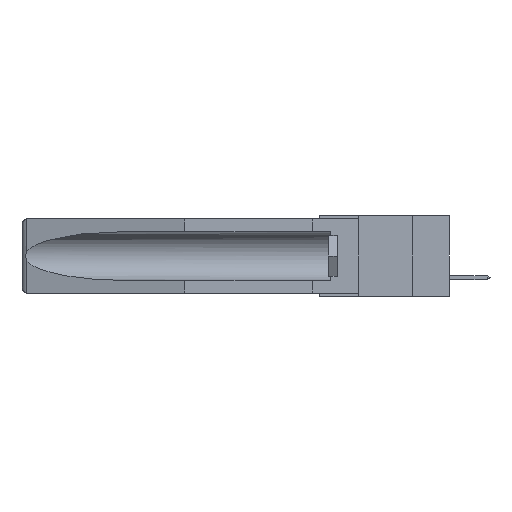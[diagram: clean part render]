
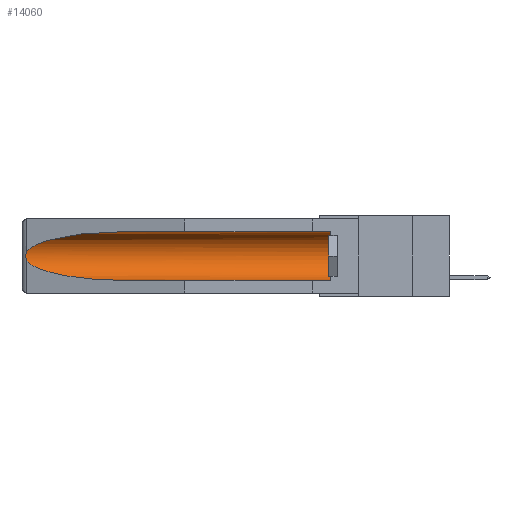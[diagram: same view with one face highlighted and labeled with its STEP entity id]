
A CAD part, left-side view. The second image highlights one B-rep face of the part: STEP entity #14060.
In plain terms, the highlighted cylindrical face has radius 2.857 mm (diameter 5.715 mm), a partial arc.
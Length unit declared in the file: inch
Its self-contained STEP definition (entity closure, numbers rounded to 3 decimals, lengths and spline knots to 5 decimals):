
#430 = EDGE_CURVE ( 'NONE', #11401, #13991, #14593, .T. ) ;
#447 = CARTESIAN_POINT ( 'NONE',  ( 0.155, -0.30754, -0.1715 ) ) ;
#508 = CARTESIAN_POINT ( 'NONE',  ( 0.155, 1.07973, -0.284 ) ) ;
#511 = EDGE_CURVE ( 'NONE', #689, #11401, #1637, .T. ) ;
#689 = VERTEX_POINT ( 'NONE', #5128 ) ;
#743 = CARTESIAN_POINT ( 'NONE',  ( 0.2675, 1.53308, -0.17534 ) ) ;
#1044 = CARTESIAN_POINT ( 'NONE',  ( 0.26537, 1.52718, -0.14972 ) ) ;
#1058 = AXIS2_PLACEMENT_3D ( 'NONE', #447, #15962, #13402 ) ;
#1455 = LINE ( 'NONE', #6484, #11748 ) ;
#1637 =( BOUNDED_CURVE ( )  B_SPLINE_CURVE ( 3, ( #12457, #15208, #7408, #1044 ),
 .UNSPECIFIED., .F., .F. ) 
 B_SPLINE_CURVE_WITH_KNOTS ( ( 4, 4 ),
 ( 4.71239, 6.08839 ),
 .UNSPECIFIED. ) 
 CURVE ( )  GEOMETRIC_REPRESENTATION_ITEM ( )  RATIONAL_B_SPLINE_CURVE ( ( 1., 0.848, 0.848, 1. ) ) 
 REPRESENTATION_ITEM ( '' )  );
#1875 = CYLINDRICAL_SURFACE ( 'NONE', #1058, 0.1125 ) ;
#2739 = DIRECTION ( 'NONE',  ( 0., 1., 0. ) ) ;
#3162 = CARTESIAN_POINT ( 'NONE',  ( 0.26537, 1.52718, -0.14972 ) ) ;
#3999 = VERTEX_POINT ( 'NONE', #508 ) ;
#4287 = FACE_OUTER_BOUND ( 'NONE', #7806, .T. ) ;
#4557 = CARTESIAN_POINT ( 'NONE',  ( 0.2673, 1.53269, -0.17917 ) ) ;
#4832 =( BOUNDED_CURVE ( )  B_SPLINE_CURVE ( 3, ( #6965, #16068, #9584, #16007 ),
 .UNSPECIFIED., .F., .F. ) 
 B_SPLINE_CURVE_WITH_KNOTS ( ( 4, 4 ),
 ( 0.1948, 1.5708 ),
 .UNSPECIFIED. ) 
 CURVE ( )  GEOMETRIC_REPRESENTATION_ITEM ( )  RATIONAL_B_SPLINE_CURVE ( ( 1., 0.848, 0.848, 1. ) ) 
 REPRESENTATION_ITEM ( '' )  );
#4895 = CARTESIAN_POINT ( 'NONE',  ( 0.155, 0.126, -0.1715 ) ) ;
#5052 = DIRECTION ( 'NONE',  ( 0., -1., 0. ) ) ;
#5128 = CARTESIAN_POINT ( 'NONE',  ( 0.155, 1.07973, -0.059 ) ) ;
#6484 = CARTESIAN_POINT ( 'NONE',  ( 0.155, -0.30754, -0.059 ) ) ;
#6965 = CARTESIAN_POINT ( 'NONE',  ( 0.26537, 1.52718, -0.19328 ) ) ;
#7408 = CARTESIAN_POINT ( 'NONE',  ( 0.25451, 1.48313, -0.09465 ) ) ;
#7496 = VERTEX_POINT ( 'NONE', #13416 ) ;
#7806 = EDGE_LOOP ( 'NONE', ( #15121, #15971, #14427, #13917, #13904, #11346 ) ) ;
#8169 = VECTOR ( 'NONE', #11522, 39.37008 ) ;
#9147 = CARTESIAN_POINT ( 'NONE',  ( 0.26537, 1.52718, -0.19328 ) ) ;
#9584 = CARTESIAN_POINT ( 'NONE',  ( 0.21114, 1.30732, -0.284 ) ) ;
#9734 = CARTESIAN_POINT ( 'NONE',  ( 0.26655, 1.53094, -0.18657 ) ) ;
#11236 = EDGE_CURVE ( 'NONE', #13269, #3999, #14902, .T. ) ;
#11346 = ORIENTED_EDGE ( 'NONE', *, *, #13916, .T. ) ;
#11401 = VERTEX_POINT ( 'NONE', #16179 ) ;
#11471 = EDGE_CURVE ( 'NONE', #13991, #3999, #4832, .T. ) ;
#11522 = DIRECTION ( 'NONE',  ( 0., 1., 0. ) ) ;
#11580 = CARTESIAN_POINT ( 'NONE',  ( 0.155, -0.30754, -0.284 ) ) ;
#11748 = VECTOR ( 'NONE', #2739, 39.37008 ) ;
#12288 = CARTESIAN_POINT ( 'NONE',  ( 0.26654, 1.53092, -0.15636 ) ) ;
#12298 = CARTESIAN_POINT ( 'NONE',  ( 0.155, 0.126, -0.284 ) ) ;
#12398 = EDGE_CURVE ( 'NONE', #13269, #7496, #13823, .T. ) ;
#12457 = CARTESIAN_POINT ( 'NONE',  ( 0.155, 1.07973, -0.059 ) ) ;
#12461 = AXIS2_PLACEMENT_3D ( 'NONE', #4895, #5052, #12693 ) ;
#12693 = DIRECTION ( 'NONE',  ( 0., 0., 1. ) ) ;
#13269 = VERTEX_POINT ( 'NONE', #12298 ) ;
#13402 = DIRECTION ( 'NONE',  ( 0., 0., 1. ) ) ;
#13416 = CARTESIAN_POINT ( 'NONE',  ( 0.155, 0.126, -0.059 ) ) ;
#13423 = CARTESIAN_POINT ( 'NONE',  ( 0.26537, 1.52718, -0.19328 ) ) ;
#13823 = CIRCLE ( 'NONE', #12461, 0.1125 ) ;
#13904 = ORIENTED_EDGE ( 'NONE', *, *, #12398, .T. ) ;
#13916 = EDGE_CURVE ( 'NONE', #7496, #689, #1455, .T. ) ;
#13917 = ORIENTED_EDGE ( 'NONE', *, *, #11236, .F. ) ;
#13991 = VERTEX_POINT ( 'NONE', #9147 ) ;
#14060 = ADVANCED_FACE ( 'NONE', ( #4287 ), #1875, .F. ) ;
#14427 = ORIENTED_EDGE ( 'NONE', *, *, #11471, .T. ) ;
#14593 = B_SPLINE_CURVE_WITH_KNOTS ( 'NONE', 3,
 ( #3162, #16049, #12288, #16107, #16160, #743, #4557, #9734, #14920, #13423 ),
 .UNSPECIFIED., .F., .F.,
 ( 4, 2, 2, 2, 4 ),
 ( 0., 0.00029, 0.00058, 0.00087, 0.00117 ),
 .UNSPECIFIED. ) ;
#14902 = LINE ( 'NONE', #11580, #8169 ) ;
#14920 = CARTESIAN_POINT ( 'NONE',  ( 0.26597, 1.5296, -0.19026 ) ) ;
#15121 = ORIENTED_EDGE ( 'NONE', *, *, #511, .T. ) ;
#15208 = CARTESIAN_POINT ( 'NONE',  ( 0.21114, 1.30732, -0.059 ) ) ;
#15962 = DIRECTION ( 'NONE',  ( 0., 1., 0. ) ) ;
#15971 = ORIENTED_EDGE ( 'NONE', *, *, #430, .T. ) ;
#16007 = CARTESIAN_POINT ( 'NONE',  ( 0.155, 1.07973, -0.284 ) ) ;
#16049 = CARTESIAN_POINT ( 'NONE',  ( 0.26597, 1.52961, -0.15275 ) ) ;
#16068 = CARTESIAN_POINT ( 'NONE',  ( 0.25451, 1.48313, -0.24835 ) ) ;
#16107 = CARTESIAN_POINT ( 'NONE',  ( 0.2673, 1.5327, -0.16383 ) ) ;
#16160 = CARTESIAN_POINT ( 'NONE',  ( 0.2675, 1.53308, -0.16763 ) ) ;
#16179 = CARTESIAN_POINT ( 'NONE',  ( 0.26537, 1.52718, -0.14972 ) ) ;
